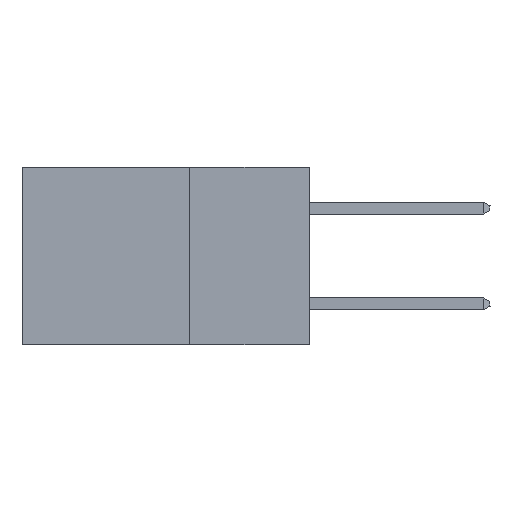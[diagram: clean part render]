
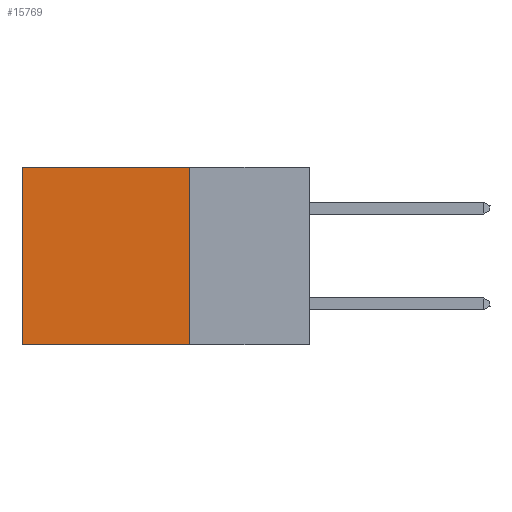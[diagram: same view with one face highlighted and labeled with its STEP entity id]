
A CAD part, left-side view. The second image highlights one B-rep face of the part: STEP entity #15769.
In plain terms, the highlighted planar face has unit normal (-1, 0, 0).
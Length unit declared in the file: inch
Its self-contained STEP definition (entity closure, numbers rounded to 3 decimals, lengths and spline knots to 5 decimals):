
#3354 = ORIENTED_EDGE ( 'NONE', *, *, #6959, .F. ) ;
#6959 = EDGE_CURVE ( 'NONE', #38687, #34054, #29633, .T. ) ;
#8869 = ORIENTED_EDGE ( 'NONE', *, *, #47091, .F. ) ;
#10368 = CARTESIAN_POINT ( 'NONE',  ( 0.2875, 0.6, -0.37 ) ) ;
#10398 = LINE ( 'NONE', #36254, #18987 ) ;
#11372 = VECTOR ( 'NONE', #46881, 39.37008 ) ;
#13284 = ORIENTED_EDGE ( 'NONE', *, *, #40378, .T. ) ;
#15769 = ADVANCED_FACE ( 'NONE', ( #25938 ), #38486, .F. ) ;
#15857 = CARTESIAN_POINT ( 'NONE',  ( 0.2875, 0.6, 0. ) ) ;
#16699 = DIRECTION ( 'NONE',  ( 1., 0., 0. ) ) ;
#18126 = DIRECTION ( 'NONE',  ( 0., 1., 0. ) ) ;
#18319 = DIRECTION ( 'NONE',  ( 0., 1., 0. ) ) ;
#18987 = VECTOR ( 'NONE', #18126, 39.37008 ) ;
#19229 = LINE ( 'NONE', #36452, #36269 ) ;
#20244 = CARTESIAN_POINT ( 'NONE',  ( 0.2875, 0.25, 0. ) ) ;
#21740 = CARTESIAN_POINT ( 'NONE',  ( 0.2875, 0.25, -0.37 ) ) ;
#23989 = ORIENTED_EDGE ( 'NONE', *, *, #27487, .T. ) ;
#25938 = FACE_OUTER_BOUND ( 'NONE', #31916, .T. ) ;
#26459 = VECTOR ( 'NONE', #41271, 39.37008 ) ;
#27487 = EDGE_CURVE ( 'NONE', #38687, #42115, #10398, .T. ) ;
#29633 = LINE ( 'NONE', #32524, #11372 ) ;
#30574 = CARTESIAN_POINT ( 'NONE',  ( 0.2875, 0.6, 0. ) ) ;
#31916 = EDGE_LOOP ( 'NONE', ( #13284, #8869, #3354, #23989 ) ) ;
#32057 = VERTEX_POINT ( 'NONE', #10368 ) ;
#32524 = CARTESIAN_POINT ( 'NONE',  ( 0.2875, 0.25, 0. ) ) ;
#34054 = VERTEX_POINT ( 'NONE', #21740 ) ;
#36254 = CARTESIAN_POINT ( 'NONE',  ( 0.2875, 0.25, 0. ) ) ;
#36269 = VECTOR ( 'NONE', #18319, 39.37008 ) ;
#36452 = CARTESIAN_POINT ( 'NONE',  ( 0.2875, 0.25, -0.37 ) ) ;
#37274 = LINE ( 'NONE', #15857, #26459 ) ;
#37472 = AXIS2_PLACEMENT_3D ( 'NONE', #20244, #16699, #42089 ) ;
#38486 = PLANE ( 'NONE',  #37472 ) ;
#38687 = VERTEX_POINT ( 'NONE', #45662 ) ;
#40378 = EDGE_CURVE ( 'NONE', #42115, #32057, #37274, .T. ) ;
#41271 = DIRECTION ( 'NONE',  ( 0., 0., -1. ) ) ;
#42089 = DIRECTION ( 'NONE',  ( 0., 0., -1. ) ) ;
#42115 = VERTEX_POINT ( 'NONE', #30574 ) ;
#45662 = CARTESIAN_POINT ( 'NONE',  ( 0.2875, 0.25, 0. ) ) ;
#46881 = DIRECTION ( 'NONE',  ( 0., 0., -1. ) ) ;
#47091 = EDGE_CURVE ( 'NONE', #34054, #32057, #19229, .T. ) ;
